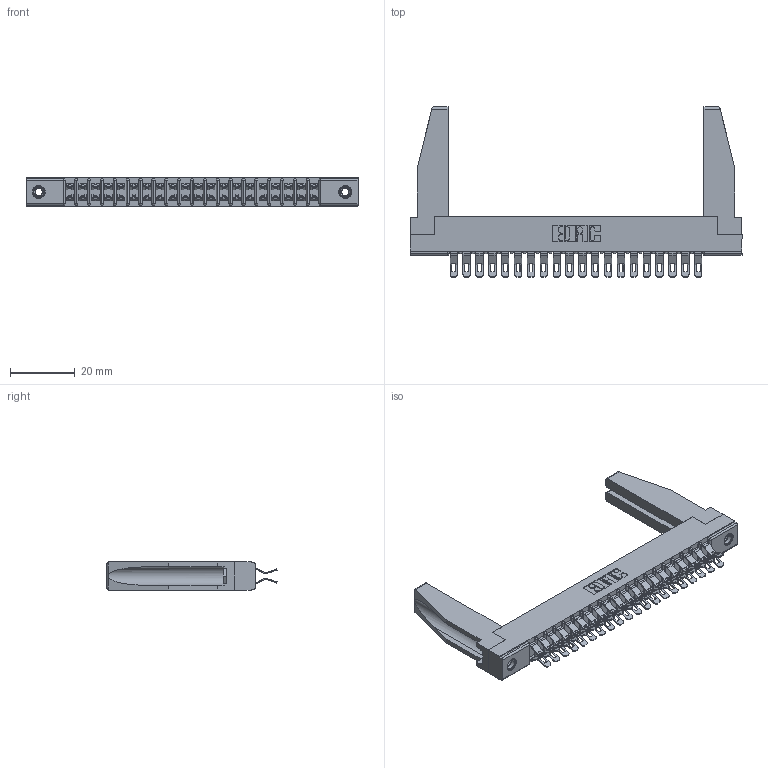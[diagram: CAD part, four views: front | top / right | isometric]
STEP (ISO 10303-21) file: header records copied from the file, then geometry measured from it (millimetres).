
FILE_DESCRIPTION (( 'STEP AP203' ), '1' );
FILE_NAME ('307-040-455-278.STEP', '2020-09-29T20:47:11', ( '' ), ( '' ), 'SwSTEP 2.0', 'SolidWorks 2020', '' );
FILE_SCHEMA (( 'CONFIG_CONTROL_DESIGN' ));
Length unit declared in the file: inch
Products named in the file (5): 307-220-078; 307-040-455-278; 345-250-001_345-250-001-102; 307-290-001_555; 307 Part_.156 Dia Mounting Holes
Assembly tree (45 placements, depth 2):
  307-040-455-278
    307 Part_.156 Dia Mounting Holes
    307-290-001_555  x40
    307-220-078  x2
    345-250-001_345-250-001-102  x2
Bounding box: 102.26 x 52.45 x 8.71 mm (x, y, z)
Volume: 10801.7 mm3; surface area: 16403.1 mm2
Topology: 45 solids, 45 shells, 2709 faces, 7893 edges, 5142 vertices
Faces by surface type: plane 1514, cylinder 1137, sphere 42, cone 12, torus 4
Entity records: 23474 total; most frequent: CARTESIAN_POINT 3862, ORIENTED_EDGE 3786, DIRECTION 3753, EDGE_CURVE 1893, LINE 1435, VECTOR 1435, VERTEX_POINT 1226, AXIS2_PLACEMENT_3D 1159
